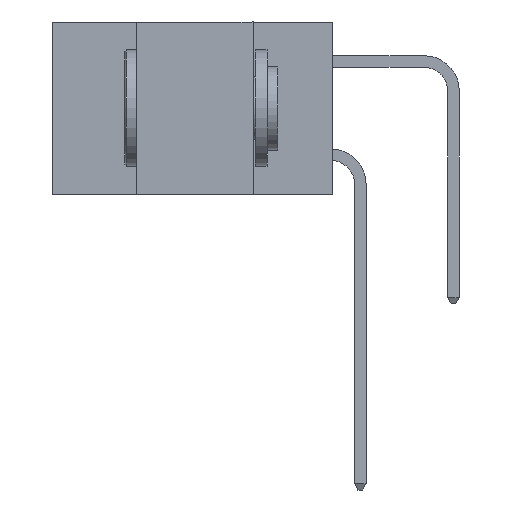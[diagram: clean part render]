
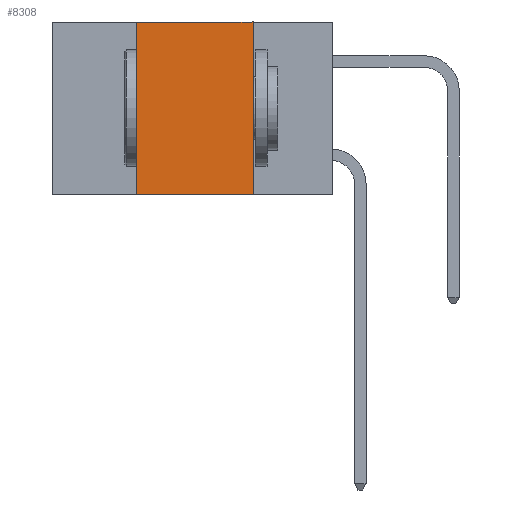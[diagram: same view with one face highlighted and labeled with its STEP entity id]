
A CAD part, left-side view. The second image highlights one B-rep face of the part: STEP entity #8308.
In plain terms, the highlighted planar face has unit normal (-1, 0, 0).
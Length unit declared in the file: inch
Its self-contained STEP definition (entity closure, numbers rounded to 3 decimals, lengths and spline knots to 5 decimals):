
#1468 = EDGE_CURVE ( 'NONE', #10075, #10340, #12039, .T. ) ;
#1929 = ORIENTED_EDGE ( 'NONE', *, *, #2586, .F. ) ;
#1954 = CARTESIAN_POINT ( 'NONE',  ( 0., 0.42, -0.37 ) ) ;
#2267 = CARTESIAN_POINT ( 'NONE',  ( 0., 0.17, -0.37 ) ) ;
#2586 = EDGE_CURVE ( 'NONE', #10340, #17251, #13534, .T. ) ;
#5611 = LINE ( 'NONE', #9622, #14116 ) ;
#7372 = EDGE_LOOP ( 'NONE', ( #1929, #19056, #15785, #8230 ) ) ;
#7746 = VECTOR ( 'NONE', #11413, 39.37008 ) ;
#8120 = CARTESIAN_POINT ( 'NONE',  ( 0., 0.6, -0.37 ) ) ;
#8230 = ORIENTED_EDGE ( 'NONE', *, *, #16323, .T. ) ;
#8308 = ADVANCED_FACE ( 'NONE', ( #17035 ), #11867, .F. ) ;
#9328 = DIRECTION ( 'NONE',  ( 0., 0., 1. ) ) ;
#9622 = CARTESIAN_POINT ( 'NONE',  ( 0., 0.42, -0.37 ) ) ;
#10075 = VERTEX_POINT ( 'NONE', #16635 ) ;
#10340 = VERTEX_POINT ( 'NONE', #11887 ) ;
#10365 = VECTOR ( 'NONE', #19389, 39.37008 ) ;
#10511 = EDGE_CURVE ( 'NONE', #15734, #10075, #5611, .T. ) ;
#10871 = LINE ( 'NONE', #8120, #10365 ) ;
#11413 = DIRECTION ( 'NONE',  ( 0., -1., 0. ) ) ;
#11480 = CARTESIAN_POINT ( 'NONE',  ( 0., 0.6, 0. ) ) ;
#11673 = DIRECTION ( 'NONE',  ( 0., 0., -1. ) ) ;
#11699 = DIRECTION ( 'NONE',  ( 1., 0., 0. ) ) ;
#11705 = CARTESIAN_POINT ( 'NONE',  ( 0., 0.6, 0. ) ) ;
#11867 = PLANE ( 'NONE',  #13059 ) ;
#11887 = CARTESIAN_POINT ( 'NONE',  ( 0., 0.17, 0. ) ) ;
#12039 = LINE ( 'NONE', #11480, #7746 ) ;
#13059 = AXIS2_PLACEMENT_3D ( 'NONE', #11705, #11699, #11673 ) ;
#13534 = LINE ( 'NONE', #20732, #14024 ) ;
#14024 = VECTOR ( 'NONE', #19102, 39.37008 ) ;
#14116 = VECTOR ( 'NONE', #9328, 39.37008 ) ;
#15734 = VERTEX_POINT ( 'NONE', #1954 ) ;
#15785 = ORIENTED_EDGE ( 'NONE', *, *, #10511, .F. ) ;
#16323 = EDGE_CURVE ( 'NONE', #15734, #17251, #10871, .T. ) ;
#16635 = CARTESIAN_POINT ( 'NONE',  ( 0., 0.42, 0. ) ) ;
#17035 = FACE_OUTER_BOUND ( 'NONE', #7372, .T. ) ;
#17251 = VERTEX_POINT ( 'NONE', #2267 ) ;
#19056 = ORIENTED_EDGE ( 'NONE', *, *, #1468, .F. ) ;
#19102 = DIRECTION ( 'NONE',  ( 0., 0., -1. ) ) ;
#19389 = DIRECTION ( 'NONE',  ( 0., -1., 0. ) ) ;
#20732 = CARTESIAN_POINT ( 'NONE',  ( 0., 0.17, -0.37 ) ) ;
